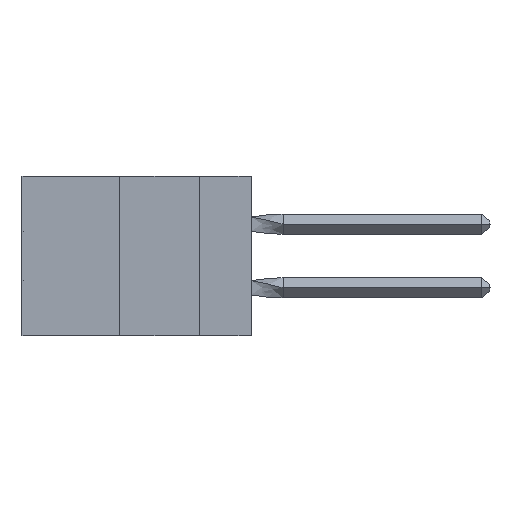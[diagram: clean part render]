
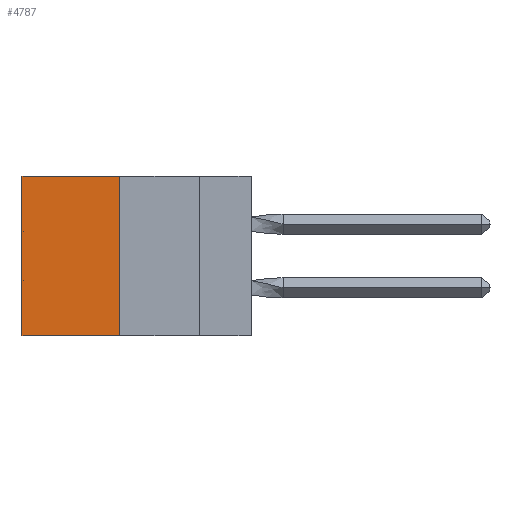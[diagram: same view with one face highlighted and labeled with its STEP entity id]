
A CAD part, left-side view. The second image highlights one B-rep face of the part: STEP entity #4787.
In plain terms, the highlighted planar face has unit normal (-1, 0, 0).
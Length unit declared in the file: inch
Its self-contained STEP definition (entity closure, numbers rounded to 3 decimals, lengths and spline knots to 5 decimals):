
#21 = LINE ( 'NONE', #22509, #14767 ) ;
#207 = CARTESIAN_POINT ( 'NONE',  ( 0.305, 0.413, -0.5 ) ) ;
#1507 = DIRECTION ( 'NONE',  ( 0., 0., -1. ) ) ;
#1944 = DIRECTION ( 'NONE',  ( 0., 1., 0. ) ) ;
#2462 = CARTESIAN_POINT ( 'NONE',  ( 0.305, 0.413, 0. ) ) ;
#2688 = CARTESIAN_POINT ( 'NONE',  ( 0.305, 0.413, -0.5 ) ) ;
#4787 = ADVANCED_FACE ( 'NONE', ( #5219 ), #21797, .F. ) ;
#5051 = VERTEX_POINT ( 'NONE', #2462 ) ;
#5219 = FACE_OUTER_BOUND ( 'NONE', #21749, .T. ) ;
#5263 = LINE ( 'NONE', #207, #23659 ) ;
#5649 = VECTOR ( 'NONE', #21645, 39.37008 ) ;
#7939 = AXIS2_PLACEMENT_3D ( 'NONE', #18885, #21504, #1507 ) ;
#10556 = CARTESIAN_POINT ( 'NONE',  ( 0.305, 0.72, 0. ) ) ;
#11314 = VERTEX_POINT ( 'NONE', #10556 ) ;
#13160 = DIRECTION ( 'NONE',  ( 0., 0., -1. ) ) ;
#14767 = VECTOR ( 'NONE', #1944, 39.37008 ) ;
#16233 = EDGE_CURVE ( 'NONE', #5051, #38668, #5263, .T. ) ;
#18016 = ORIENTED_EDGE ( 'NONE', *, *, #16233, .F. ) ;
#18218 = EDGE_CURVE ( 'NONE', #38668, #28716, #31455, .T. ) ;
#18257 = ORIENTED_EDGE ( 'NONE', *, *, #18218, .F. ) ;
#18885 = CARTESIAN_POINT ( 'NONE',  ( 0.305, 0.413, -0.5 ) ) ;
#19240 = ORIENTED_EDGE ( 'NONE', *, *, #21856, .T. ) ;
#19268 = VECTOR ( 'NONE', #13160, 39.37008 ) ;
#21504 = DIRECTION ( 'NONE',  ( 1., 0., 0. ) ) ;
#21645 = DIRECTION ( 'NONE',  ( 0., 1., 0. ) ) ;
#21749 = EDGE_LOOP ( 'NONE', ( #25860, #18257, #18016, #19240 ) ) ;
#21797 = PLANE ( 'NONE',  #7939 ) ;
#21856 = EDGE_CURVE ( 'NONE', #5051, #11314, #21, .T. ) ;
#22509 = CARTESIAN_POINT ( 'NONE',  ( 0.305, 0.413, 0. ) ) ;
#23659 = VECTOR ( 'NONE', #23740, 39.37008 ) ;
#23740 = DIRECTION ( 'NONE',  ( 0., 0., -1. ) ) ;
#24907 = CARTESIAN_POINT ( 'NONE',  ( 0.305, 0.72, -0.5 ) ) ;
#25860 = ORIENTED_EDGE ( 'NONE', *, *, #32528, .T. ) ;
#26064 = LINE ( 'NONE', #26659, #19268 ) ;
#26659 = CARTESIAN_POINT ( 'NONE',  ( 0.305, 0.72, -0.5 ) ) ;
#28716 = VERTEX_POINT ( 'NONE', #24907 ) ;
#31455 = LINE ( 'NONE', #41810, #5649 ) ;
#32528 = EDGE_CURVE ( 'NONE', #11314, #28716, #26064, .T. ) ;
#38668 = VERTEX_POINT ( 'NONE', #2688 ) ;
#41810 = CARTESIAN_POINT ( 'NONE',  ( 0.305, 0.413, -0.5 ) ) ;
